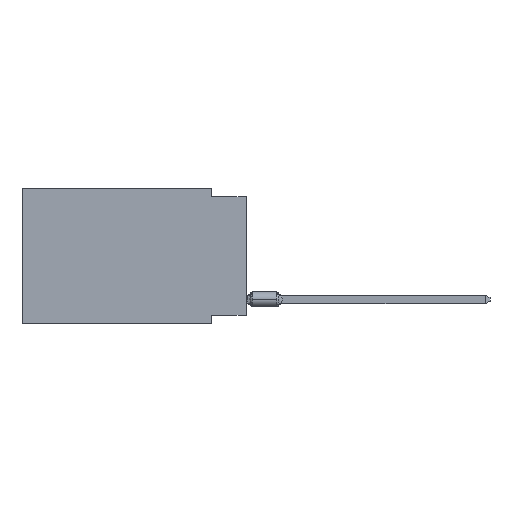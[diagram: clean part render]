
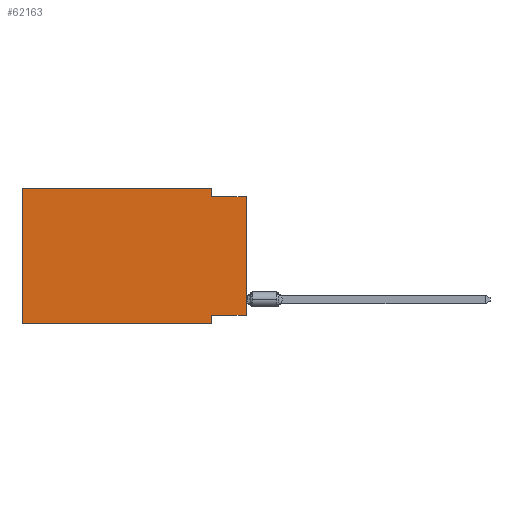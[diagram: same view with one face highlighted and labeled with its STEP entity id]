
A CAD part, left-side view. The second image highlights one B-rep face of the part: STEP entity #62163.
In plain terms, the highlighted planar face has unit normal (-1, 0, 0).
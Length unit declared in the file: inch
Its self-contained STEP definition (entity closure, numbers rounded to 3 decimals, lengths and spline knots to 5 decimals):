
#220 = VECTOR ( 'NONE', #62918, 39.37008 ) ;
#866 = ORIENTED_EDGE ( 'NONE', *, *, #55108, .T. ) ;
#3444 = EDGE_CURVE ( 'NONE', #33097, #52081, #57001, .T. ) ;
#4139 = AXIS2_PLACEMENT_3D ( 'NONE', #16229, #62441, #10535 ) ;
#5116 = EDGE_CURVE ( 'NONE', #33416, #5461, #58941, .T. ) ;
#5461 = VERTEX_POINT ( 'NONE', #23364 ) ;
#9690 = DIRECTION ( 'NONE',  ( 0., -1., 0. ) ) ;
#10346 = VECTOR ( 'NONE', #48543, 39.37008 ) ;
#10535 = DIRECTION ( 'NONE',  ( 0., 0., -1. ) ) ;
#11661 = LINE ( 'NONE', #22062, #220 ) ;
#12900 = DIRECTION ( 'NONE',  ( 0., 0., -1. ) ) ;
#13260 = EDGE_CURVE ( 'NONE', #5461, #33097, #38364, .T. ) ;
#14727 = LINE ( 'NONE', #55585, #42897 ) ;
#16229 = CARTESIAN_POINT ( 'NONE',  ( 0., 0.645, 0. ) ) ;
#16371 = EDGE_CURVE ( 'NONE', #17758, #35288, #54219, .T. ) ;
#17395 = CARTESIAN_POINT ( 'NONE',  ( 0., 0.1, -0.39 ) ) ;
#17600 = VECTOR ( 'NONE', #12900, 39.37008 ) ;
#17758 = VERTEX_POINT ( 'NONE', #54565 ) ;
#17861 = LINE ( 'NONE', #32945, #21616 ) ;
#19131 = DIRECTION ( 'NONE',  ( 0., 1., 0. ) ) ;
#19278 = ORIENTED_EDGE ( 'NONE', *, *, #3444, .F. ) ;
#20623 = ORIENTED_EDGE ( 'NONE', *, *, #64555, .F. ) ;
#21314 = VECTOR ( 'NONE', #47314, 39.37008 ) ;
#21616 = VECTOR ( 'NONE', #48686, 39.37008 ) ;
#22062 = CARTESIAN_POINT ( 'NONE',  ( 0., 0., 0. ) ) ;
#22069 = EDGE_CURVE ( 'NONE', #51102, #33416, #17861, .T. ) ;
#22420 = EDGE_CURVE ( 'NONE', #33522, #52081, #11661, .T. ) ;
#22854 = LINE ( 'NONE', #23843, #38579 ) ;
#23364 = CARTESIAN_POINT ( 'NONE',  ( 0., 0.1, 0. ) ) ;
#23784 = CARTESIAN_POINT ( 'NONE',  ( 0., 0.645, 0. ) ) ;
#23843 = CARTESIAN_POINT ( 'NONE',  ( 0., 0., -0.365 ) ) ;
#25826 = EDGE_LOOP ( 'NONE', ( #29365, #19278, #57378, #52299, #27472, #866, #42441, #20623 ) ) ;
#26897 = CARTESIAN_POINT ( 'NONE',  ( 0., 0., -0.025 ) ) ;
#26940 = CARTESIAN_POINT ( 'NONE',  ( 0., 0., -0.365 ) ) ;
#26948 = CARTESIAN_POINT ( 'NONE',  ( 0., 0.645, -0.39 ) ) ;
#27472 = ORIENTED_EDGE ( 'NONE', *, *, #22069, .F. ) ;
#29365 = ORIENTED_EDGE ( 'NONE', *, *, #22420, .T. ) ;
#29675 = CARTESIAN_POINT ( 'NONE',  ( 0., 0., -0.025 ) ) ;
#32846 = DIRECTION ( 'NONE',  ( 0., -1., 0. ) ) ;
#32945 = CARTESIAN_POINT ( 'NONE',  ( 0., 0.645, 0. ) ) ;
#33097 = VERTEX_POINT ( 'NONE', #33587 ) ;
#33416 = VERTEX_POINT ( 'NONE', #60432 ) ;
#33522 = VERTEX_POINT ( 'NONE', #26940 ) ;
#33587 = CARTESIAN_POINT ( 'NONE',  ( 0., 0.1, -0.025 ) ) ;
#35288 = VERTEX_POINT ( 'NONE', #53311 ) ;
#36439 = VECTOR ( 'NONE', #32846, 39.37008 ) ;
#38364 = LINE ( 'NONE', #49070, #17600 ) ;
#38579 = VECTOR ( 'NONE', #19131, 39.37008 ) ;
#39812 = FACE_OUTER_BOUND ( 'NONE', #25826, .T. ) ;
#42441 = ORIENTED_EDGE ( 'NONE', *, *, #16371, .F. ) ;
#42897 = VECTOR ( 'NONE', #9690, 39.37008 ) ;
#47314 = DIRECTION ( 'NONE',  ( 0., -1., 0. ) ) ;
#48543 = DIRECTION ( 'NONE',  ( 0., 0., -1. ) ) ;
#48686 = DIRECTION ( 'NONE',  ( 0., 0., 1. ) ) ;
#49070 = CARTESIAN_POINT ( 'NONE',  ( 0., 0.1, 0. ) ) ;
#51102 = VERTEX_POINT ( 'NONE', #26948 ) ;
#52081 = VERTEX_POINT ( 'NONE', #29675 ) ;
#52299 = ORIENTED_EDGE ( 'NONE', *, *, #5116, .F. ) ;
#53311 = CARTESIAN_POINT ( 'NONE',  ( 0., 0.1, -0.39 ) ) ;
#54219 = LINE ( 'NONE', #17395, #10346 ) ;
#54565 = CARTESIAN_POINT ( 'NONE',  ( 0., 0.1, -0.365 ) ) ;
#55108 = EDGE_CURVE ( 'NONE', #51102, #35288, #14727, .T. ) ;
#55202 = PLANE ( 'NONE',  #4139 ) ;
#55585 = CARTESIAN_POINT ( 'NONE',  ( 0., 0.645, -0.39 ) ) ;
#57001 = LINE ( 'NONE', #26897, #21314 ) ;
#57378 = ORIENTED_EDGE ( 'NONE', *, *, #13260, .F. ) ;
#58941 = LINE ( 'NONE', #23784, #36439 ) ;
#60432 = CARTESIAN_POINT ( 'NONE',  ( 0., 0.645, 0. ) ) ;
#62163 = ADVANCED_FACE ( 'NONE', ( #39812 ), #55202, .F. ) ;
#62441 = DIRECTION ( 'NONE',  ( 1., 0., 0. ) ) ;
#62918 = DIRECTION ( 'NONE',  ( 0., 0., 1. ) ) ;
#64555 = EDGE_CURVE ( 'NONE', #33522, #17758, #22854, .T. ) ;
